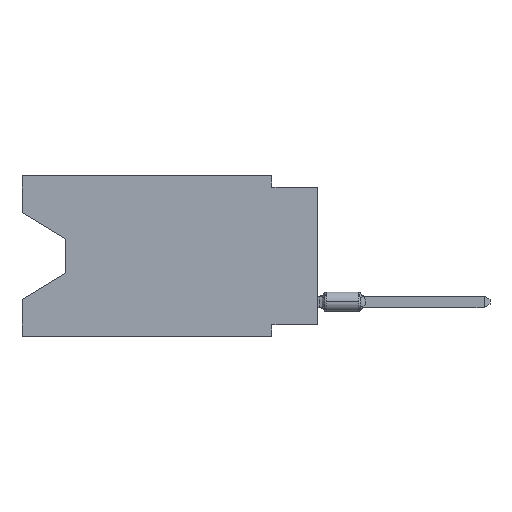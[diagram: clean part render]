
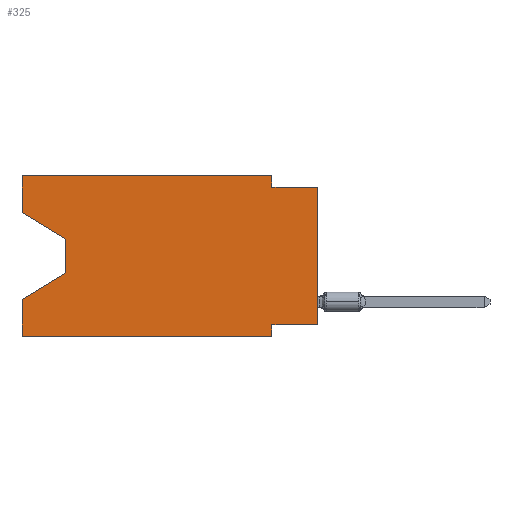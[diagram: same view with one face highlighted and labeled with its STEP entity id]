
A CAD part, left-side view. The second image highlights one B-rep face of the part: STEP entity #325.
In plain terms, the highlighted planar face has unit normal (-1, 0, 0).
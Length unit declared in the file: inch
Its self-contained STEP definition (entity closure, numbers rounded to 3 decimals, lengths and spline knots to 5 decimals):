
#41 = LINE ( 'NONE', #7923, #4916 ) ;
#184 = EDGE_CURVE ( 'NONE', #10621, #11912, #5319, .T. ) ;
#227 = CARTESIAN_POINT ( 'NONE',  ( 0., 0.645, 0. ) ) ;
#325 = ADVANCED_FACE ( 'NONE', ( #1803 ), #14798, .F. ) ;
#540 = EDGE_CURVE ( 'NONE', #12071, #6475, #13790, .T. ) ;
#595 = DIRECTION ( 'NONE',  ( 0., 0., 1. ) ) ;
#1577 = ORIENTED_EDGE ( 'NONE', *, *, #13840, .T. ) ;
#1704 = DIRECTION ( 'NONE',  ( 0., 0., -1. ) ) ;
#1801 = ORIENTED_EDGE ( 'NONE', *, *, #16033, .T. ) ;
#1803 = FACE_OUTER_BOUND ( 'NONE', #16456, .T. ) ;
#1883 = CARTESIAN_POINT ( 'NONE',  ( 0., 0.55, -0.212 ) ) ;
#1972 = VECTOR ( 'NONE', #2296, 39.37008 ) ;
#2081 = EDGE_CURVE ( 'NONE', #13888, #3758, #5040, .T. ) ;
#2088 = CARTESIAN_POINT ( 'NONE',  ( 0., 0., -0.325 ) ) ;
#2296 = DIRECTION ( 'NONE',  ( 0., -1., 0. ) ) ;
#2356 = EDGE_CURVE ( 'NONE', #10306, #6475, #13246, .T. ) ;
#2505 = EDGE_CURVE ( 'NONE', #14151, #10306, #16183, .T. ) ;
#2940 = CARTESIAN_POINT ( 'NONE',  ( 0., 0.645, -0.26975 ) ) ;
#3138 = DIRECTION ( 'NONE',  ( 1., 0., 0. ) ) ;
#3278 = EDGE_CURVE ( 'NONE', #10631, #16549, #10295, .T. ) ;
#3758 = VERTEX_POINT ( 'NONE', #1883 ) ;
#4003 = LINE ( 'NONE', #9112, #13242 ) ;
#4092 = DIRECTION ( 'NONE',  ( 0., -1., 0. ) ) ;
#4182 = VERTEX_POINT ( 'NONE', #4302 ) ;
#4183 = CARTESIAN_POINT ( 'NONE',  ( 0., 0., -0.025 ) ) ;
#4253 = DIRECTION ( 'NONE',  ( 0., 0., 1. ) ) ;
#4302 = CARTESIAN_POINT ( 'NONE',  ( 0., 0.1, 0. ) ) ;
#4350 = CARTESIAN_POINT ( 'NONE',  ( 0., 0.1, -0.35 ) ) ;
#4616 = EDGE_CURVE ( 'NONE', #12071, #6995, #11825, .T. ) ;
#4683 = DIRECTION ( 'NONE',  ( 0., 1., 0. ) ) ;
#4794 = CARTESIAN_POINT ( 'NONE',  ( 0., 0.55, -0.138 ) ) ;
#4801 = CARTESIAN_POINT ( 'NONE',  ( 0., 0.55, -0.212 ) ) ;
#4916 = VECTOR ( 'NONE', #11778, 39.37008 ) ;
#5040 = LINE ( 'NONE', #4794, #13541 ) ;
#5273 = VECTOR ( 'NONE', #8654, 39.37008 ) ;
#5319 = LINE ( 'NONE', #227, #12181 ) ;
#5432 = EDGE_CURVE ( 'NONE', #4182, #10631, #9496, .T. ) ;
#5477 = VECTOR ( 'NONE', #595, 39.37008 ) ;
#5824 = CARTESIAN_POINT ( 'NONE',  ( 0., 0., -0.325 ) ) ;
#6475 = VERTEX_POINT ( 'NONE', #9781 ) ;
#6551 = CARTESIAN_POINT ( 'NONE',  ( 0., 0.645, -0.08025 ) ) ;
#6942 = ORIENTED_EDGE ( 'NONE', *, *, #2505, .F. ) ;
#6987 = CARTESIAN_POINT ( 'NONE',  ( 0., 0.1, 0. ) ) ;
#6995 = VERTEX_POINT ( 'NONE', #2940 ) ;
#7282 = LINE ( 'NONE', #14834, #15965 ) ;
#7551 = DIRECTION ( 'NONE',  ( 0., 0., -1. ) ) ;
#7679 = VECTOR ( 'NONE', #4092, 39.37008 ) ;
#7923 = CARTESIAN_POINT ( 'NONE',  ( 0., 0.645, 0. ) ) ;
#8033 = CARTESIAN_POINT ( 'NONE',  ( 0., 0., -0.025 ) ) ;
#8145 = VECTOR ( 'NONE', #1704, 39.37008 ) ;
#8226 = ORIENTED_EDGE ( 'NONE', *, *, #10195, .F. ) ;
#8392 = CARTESIAN_POINT ( 'NONE',  ( 0., 0.645, -0.35 ) ) ;
#8620 = DIRECTION ( 'NONE',  ( 0., -0.855, -0.519 ) ) ;
#8654 = DIRECTION ( 'NONE',  ( 0., 0.855, -0.519 ) ) ;
#8760 = CARTESIAN_POINT ( 'NONE',  ( 0., 0.645, -0.35 ) ) ;
#9112 = CARTESIAN_POINT ( 'NONE',  ( 0., 0., 0. ) ) ;
#9117 = CARTESIAN_POINT ( 'NONE',  ( 0., 0.55, -0.138 ) ) ;
#9137 = ORIENTED_EDGE ( 'NONE', *, *, #184, .F. ) ;
#9491 = AXIS2_PLACEMENT_3D ( 'NONE', #9749, #3138, #12106 ) ;
#9496 = LINE ( 'NONE', #6987, #8145 ) ;
#9537 = ORIENTED_EDGE ( 'NONE', *, *, #2356, .F. ) ;
#9749 = CARTESIAN_POINT ( 'NONE',  ( 0., 0.645, 0. ) ) ;
#9781 = CARTESIAN_POINT ( 'NONE',  ( 0., 0.1, -0.35 ) ) ;
#10195 = EDGE_CURVE ( 'NONE', #11912, #4182, #41, .T. ) ;
#10295 = LINE ( 'NONE', #8033, #7679 ) ;
#10306 = VERTEX_POINT ( 'NONE', #14143 ) ;
#10484 = CARTESIAN_POINT ( 'NONE',  ( 0., 0.1, -0.025 ) ) ;
#10621 = VERTEX_POINT ( 'NONE', #6551 ) ;
#10631 = VERTEX_POINT ( 'NONE', #10484 ) ;
#10733 = CARTESIAN_POINT ( 'NONE',  ( 0., 0.645, 0. ) ) ;
#10917 = ORIENTED_EDGE ( 'NONE', *, *, #5432, .F. ) ;
#11044 = EDGE_CURVE ( 'NONE', #14151, #16549, #4003, .T. ) ;
#11596 = ORIENTED_EDGE ( 'NONE', *, *, #4616, .F. ) ;
#11778 = DIRECTION ( 'NONE',  ( 0., -1., 0. ) ) ;
#11825 = LINE ( 'NONE', #10733, #5477 ) ;
#11906 = DIRECTION ( 'NONE',  ( 0., 0., -1. ) ) ;
#11912 = VERTEX_POINT ( 'NONE', #14202 ) ;
#12071 = VERTEX_POINT ( 'NONE', #8392 ) ;
#12106 = DIRECTION ( 'NONE',  ( 0., 0., -1. ) ) ;
#12181 = VECTOR ( 'NONE', #14303, 39.37008 ) ;
#12221 = ORIENTED_EDGE ( 'NONE', *, *, #11044, .T. ) ;
#12728 = VECTOR ( 'NONE', #4683, 39.37008 ) ;
#13242 = VECTOR ( 'NONE', #4253, 39.37008 ) ;
#13246 = LINE ( 'NONE', #4350, #14357 ) ;
#13541 = VECTOR ( 'NONE', #7551, 39.37008 ) ;
#13790 = LINE ( 'NONE', #8760, #1972 ) ;
#13840 = EDGE_CURVE ( 'NONE', #10621, #13888, #7282, .T. ) ;
#13888 = VERTEX_POINT ( 'NONE', #9117 ) ;
#14143 = CARTESIAN_POINT ( 'NONE',  ( 0., 0.1, -0.325 ) ) ;
#14151 = VERTEX_POINT ( 'NONE', #5824 ) ;
#14202 = CARTESIAN_POINT ( 'NONE',  ( 0., 0.645, 0. ) ) ;
#14303 = DIRECTION ( 'NONE',  ( 0., 0., 1. ) ) ;
#14357 = VECTOR ( 'NONE', #11906, 39.37008 ) ;
#14516 = ORIENTED_EDGE ( 'NONE', *, *, #2081, .T. ) ;
#14798 = PLANE ( 'NONE',  #9491 ) ;
#14834 = CARTESIAN_POINT ( 'NONE',  ( 0., 0.645, -0.08025 ) ) ;
#14969 = ORIENTED_EDGE ( 'NONE', *, *, #540, .T. ) ;
#15965 = VECTOR ( 'NONE', #8620, 39.37008 ) ;
#16033 = EDGE_CURVE ( 'NONE', #3758, #6995, #16307, .T. ) ;
#16183 = LINE ( 'NONE', #2088, #12728 ) ;
#16247 = ORIENTED_EDGE ( 'NONE', *, *, #3278, .F. ) ;
#16307 = LINE ( 'NONE', #4801, #5273 ) ;
#16456 = EDGE_LOOP ( 'NONE', ( #1577, #14516, #1801, #11596, #14969, #9537, #6942, #12221, #16247, #10917, #8226, #9137 ) ) ;
#16549 = VERTEX_POINT ( 'NONE', #4183 ) ;
